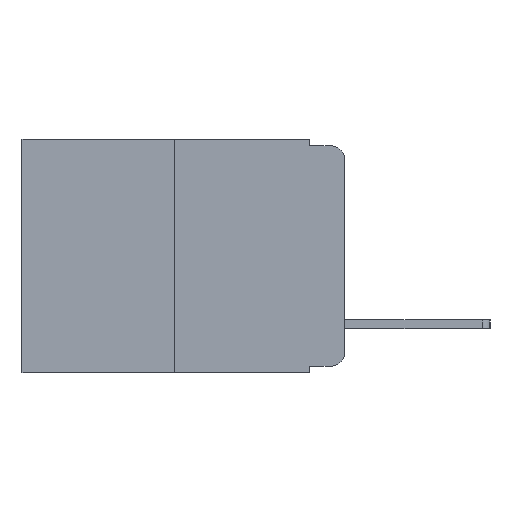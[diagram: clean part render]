
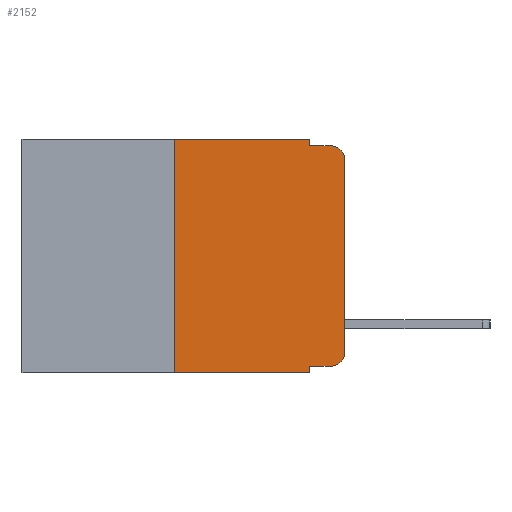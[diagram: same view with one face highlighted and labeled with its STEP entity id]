
A CAD part, left-side view. The second image highlights one B-rep face of the part: STEP entity #2152.
In plain terms, the highlighted planar face has unit normal (-1, 0, 0).
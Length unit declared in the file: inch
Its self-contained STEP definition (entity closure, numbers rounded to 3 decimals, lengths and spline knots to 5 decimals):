
#615 = LINE ( 'NONE', #11892, #10585 ) ;
#709 = CARTESIAN_POINT ( 'NONE',  ( 0., 0.25, 0. ) ) ;
#712 = LINE ( 'NONE', #11812, #8238 ) ;
#812 = LINE ( 'NONE', #1240, #10770 ) ;
#1153 = VERTEX_POINT ( 'NONE', #7216 ) ;
#1240 = CARTESIAN_POINT ( 'NONE',  ( 0., 0.051, 0. ) ) ;
#1351 = EDGE_CURVE ( 'NONE', #8405, #8167, #3370, .T. ) ;
#1452 = FACE_OUTER_BOUND ( 'NONE', #3701, .T. ) ;
#1778 = EDGE_CURVE ( 'NONE', #5568, #6472, #9021, .T. ) ;
#2008 = ORIENTED_EDGE ( 'NONE', *, *, #5119, .F. ) ;
#2152 = ADVANCED_FACE ( 'NONE', ( #1452 ), #8924, .F. ) ;
#2330 = VECTOR ( 'NONE', #11188, 39.37008 ) ;
#2471 = EDGE_CURVE ( 'NONE', #4092, #5568, #615, .T. ) ;
#2613 = DIRECTION ( 'NONE',  ( -1., 0., 0. ) ) ;
#2686 = CARTESIAN_POINT ( 'NONE',  ( 0., 0.051, -0.343 ) ) ;
#2694 = DIRECTION ( 'NONE',  ( 0., 0., -1. ) ) ;
#2747 = VECTOR ( 'NONE', #8404, 39.37008 ) ;
#2754 = CARTESIAN_POINT ( 'NONE',  ( 0., 0.051, 0. ) ) ;
#2862 = DIRECTION ( 'NONE',  ( 1., 0., 0. ) ) ;
#2947 = VERTEX_POINT ( 'NONE', #4855 ) ;
#2971 = ORIENTED_EDGE ( 'NONE', *, *, #2471, .T. ) ;
#3130 = EDGE_CURVE ( 'NONE', #4092, #9579, #11593, .T. ) ;
#3290 = ORIENTED_EDGE ( 'NONE', *, *, #1778, .T. ) ;
#3370 = LINE ( 'NONE', #3604, #8155 ) ;
#3531 = CARTESIAN_POINT ( 'NONE',  ( 0., 0.473, 0. ) ) ;
#3604 = CARTESIAN_POINT ( 'NONE',  ( 0., 0.473, 0. ) ) ;
#3701 = EDGE_LOOP ( 'NONE', ( #6012, #3744, #8802, #11544, #4391, #2008, #12408, #7776, #2971, #3290 ) ) ;
#3744 = ORIENTED_EDGE ( 'NONE', *, *, #8903, .T. ) ;
#3807 = VECTOR ( 'NONE', #7307, 39.37008 ) ;
#4092 = VERTEX_POINT ( 'NONE', #4563 ) ;
#4245 = CARTESIAN_POINT ( 'NONE',  ( 0., 0., -0.313 ) ) ;
#4274 = CIRCLE ( 'NONE', #12071, 0.02 ) ;
#4391 = ORIENTED_EDGE ( 'NONE', *, *, #1351, .F. ) ;
#4563 = CARTESIAN_POINT ( 'NONE',  ( 0., 0.051, -0.333 ) ) ;
#4855 = CARTESIAN_POINT ( 'NONE',  ( 0., 0., -0.03 ) ) ;
#4979 = LINE ( 'NONE', #10261, #2330 ) ;
#5119 = EDGE_CURVE ( 'NONE', #8270, #8405, #712, .T. ) ;
#5156 = AXIS2_PLACEMENT_3D ( 'NONE', #10691, #10592, #10589 ) ;
#5552 = DIRECTION ( 'NONE',  ( 0., -1., 0. ) ) ;
#5568 = VERTEX_POINT ( 'NONE', #8730 ) ;
#5755 = EDGE_CURVE ( 'NONE', #8167, #10165, #812, .T. ) ;
#6012 = ORIENTED_EDGE ( 'NONE', *, *, #10735, .T. ) ;
#6222 = DIRECTION ( 'NONE',  ( 0., 0., 1. ) ) ;
#6340 = CARTESIAN_POINT ( 'NONE',  ( 0., 0.473, -0.343 ) ) ;
#6472 = VERTEX_POINT ( 'NONE', #4245 ) ;
#7216 = CARTESIAN_POINT ( 'NONE',  ( 0., 0.02, -0.01 ) ) ;
#7307 = DIRECTION ( 'NONE',  ( 0., -1., 0. ) ) ;
#7440 = CARTESIAN_POINT ( 'NONE',  ( 0., 0.051, -0.01 ) ) ;
#7644 = EDGE_CURVE ( 'NONE', #10165, #1153, #7847, .T. ) ;
#7776 = ORIENTED_EDGE ( 'NONE', *, *, #3130, .F. ) ;
#7847 = LINE ( 'NONE', #7440, #2747 ) ;
#8082 = AXIS2_PLACEMENT_3D ( 'NONE', #3531, #2862, #8565 ) ;
#8155 = VECTOR ( 'NONE', #5552, 39.37008 ) ;
#8167 = VERTEX_POINT ( 'NONE', #11890 ) ;
#8210 = EDGE_CURVE ( 'NONE', #8270, #9579, #11300, .T. ) ;
#8238 = VECTOR ( 'NONE', #6222, 39.37008 ) ;
#8270 = VERTEX_POINT ( 'NONE', #8347 ) ;
#8347 = CARTESIAN_POINT ( 'NONE',  ( 0., 0.25, -0.343 ) ) ;
#8376 = CARTESIAN_POINT ( 'NONE',  ( 0., 0.02, -0.03 ) ) ;
#8404 = DIRECTION ( 'NONE',  ( 0., -1., 0. ) ) ;
#8405 = VERTEX_POINT ( 'NONE', #709 ) ;
#8565 = DIRECTION ( 'NONE',  ( 0., 0., -1. ) ) ;
#8730 = CARTESIAN_POINT ( 'NONE',  ( 0., 0.02, -0.333 ) ) ;
#8802 = ORIENTED_EDGE ( 'NONE', *, *, #7644, .F. ) ;
#8903 = EDGE_CURVE ( 'NONE', #2947, #1153, #4274, .T. ) ;
#8924 = PLANE ( 'NONE',  #8082 ) ;
#9021 = CIRCLE ( 'NONE', #5156, 0.02 ) ;
#9292 = DIRECTION ( 'NONE',  ( 0., 0., -1. ) ) ;
#9579 = VERTEX_POINT ( 'NONE', #2686 ) ;
#10165 = VERTEX_POINT ( 'NONE', #11275 ) ;
#10261 = CARTESIAN_POINT ( 'NONE',  ( 0., 0., 0. ) ) ;
#10585 = VECTOR ( 'NONE', #11197, 39.37008 ) ;
#10589 = DIRECTION ( 'NONE',  ( 0., 0., -1. ) ) ;
#10592 = DIRECTION ( 'NONE',  ( -1., 0., 0. ) ) ;
#10691 = CARTESIAN_POINT ( 'NONE',  ( 0., 0.02, -0.313 ) ) ;
#10735 = EDGE_CURVE ( 'NONE', #6472, #2947, #4979, .T. ) ;
#10770 = VECTOR ( 'NONE', #11798, 39.37008 ) ;
#11188 = DIRECTION ( 'NONE',  ( 0., 0., 1. ) ) ;
#11197 = DIRECTION ( 'NONE',  ( 0., -1., 0. ) ) ;
#11275 = CARTESIAN_POINT ( 'NONE',  ( 0., 0.051, -0.01 ) ) ;
#11296 = VECTOR ( 'NONE', #2694, 39.37008 ) ;
#11300 = LINE ( 'NONE', #6340, #3807 ) ;
#11544 = ORIENTED_EDGE ( 'NONE', *, *, #5755, .F. ) ;
#11593 = LINE ( 'NONE', #2754, #11296 ) ;
#11798 = DIRECTION ( 'NONE',  ( 0., 0., -1. ) ) ;
#11812 = CARTESIAN_POINT ( 'NONE',  ( 0., 0.25, 0. ) ) ;
#11890 = CARTESIAN_POINT ( 'NONE',  ( 0., 0.051, 0. ) ) ;
#11892 = CARTESIAN_POINT ( 'NONE',  ( 0., 0.051, -0.333 ) ) ;
#12071 = AXIS2_PLACEMENT_3D ( 'NONE', #8376, #2613, #9292 ) ;
#12408 = ORIENTED_EDGE ( 'NONE', *, *, #8210, .T. ) ;
